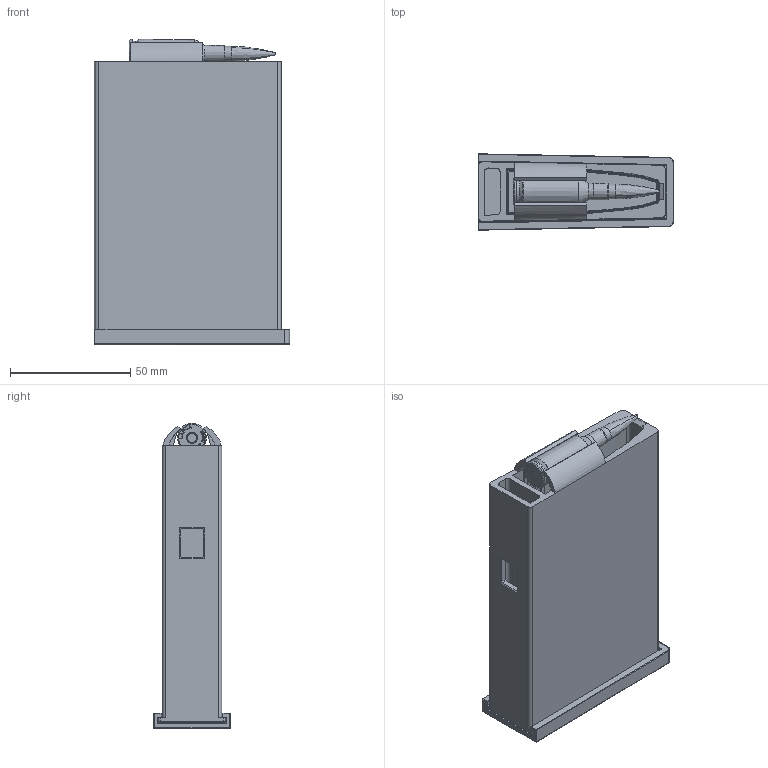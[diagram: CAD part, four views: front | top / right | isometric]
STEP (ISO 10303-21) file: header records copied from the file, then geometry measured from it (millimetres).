
FILE_DESCRIPTION(/* description */ (''),/* implementation_level */ '2;1');
FILE_NAME(/* name */ 'aics_magazine_6mm_br.step',/* time_stamp */ '2023-11-22T08:52:41+13:00',/* author */ (''),/* organization */ (''),/* preprocessor_version */ 'ST-DEVELOPER v20',/* originating_system */ 'Autodesk Translation Framework v12.14.0.127',/* authorisation */ '');
FILE_SCHEMA (('AUTOMOTIVE_DESIGN { 1 0 10303 214 3 1 1 }'));
Length unit declared in the file: millimetre
Products named in the file (5): aics_magazine; 6mmbr_assembled; 6mmbr brass; berger_109gr_long_range_hybrid; cci450
Assembly tree (4 placements, depth 3):
  aics_magazine
    6mmbr_assembled
      6mmbr brass
      berger_109gr_long_range_hybrid
      cci450
Bounding box: 81 x 31.69 x 126.81 mm (x, y, z)
Volume: 85033.1 mm3; surface area: 66087.4 mm2
Topology: 7 solids, 7 shells, 721 faces, 1840 edges, 1165 vertices
Faces by surface type: plane 334, bspline 200, cylinder 150, torus 14, sphere 13, cone 10
Full cylindrical faces by diameter (mm): 1.5 x1, 3.175 x1, 4.445 x1, 4.45 x1, 6.171 x1, 6.172 x1, 10 x1, 10.39 x1, 11 x1, 12.01 x1
Entity records: 28731 total; most frequent: CARTESIAN_POINT 12389, ORIENTED_EDGE 3680, DIRECTION 2758, EDGE_CURVE 1840, VERTEX_POINT 1165, LINE 1136, VECTOR 1136, AXIS2_PLACEMENT_3D 811
